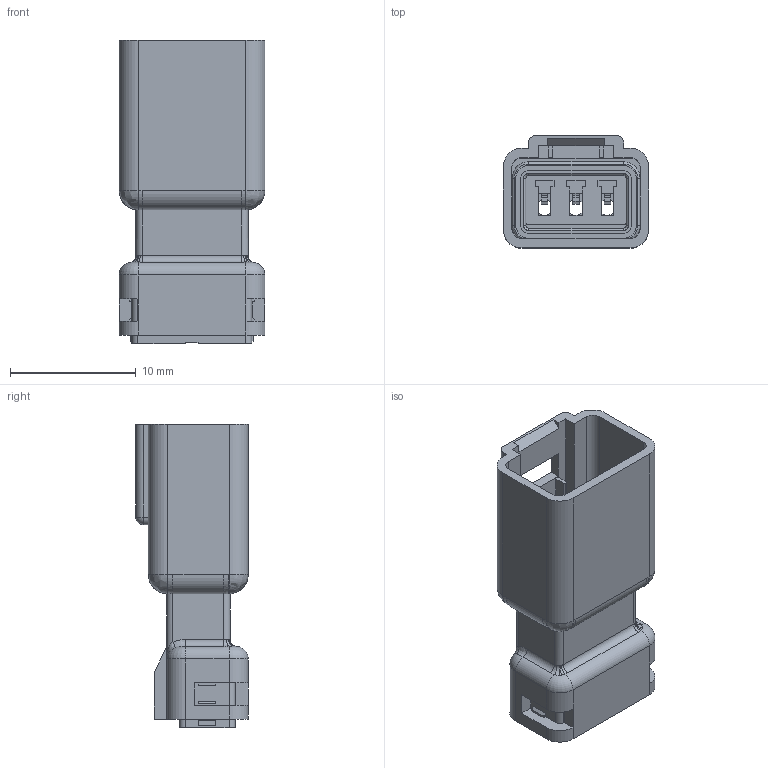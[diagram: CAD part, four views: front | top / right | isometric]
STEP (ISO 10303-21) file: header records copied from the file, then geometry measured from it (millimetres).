
FILE_DESCRIPTION (( 'STEP AP214' ), '1' );
FILE_NAME ('565-003-000-311.STEP', '2020-07-27T15:17:34', ( '' ), ( '' ), 'SwSTEP 2.0', 'SolidWorks 2020', '' );
FILE_SCHEMA (( 'AUTOMOTIVE_DESIGN' ));
Length unit declared in the file: millimetre
Products named in the file (5): 565-003-000-311_Front Gasket; 565-003-000-311; 565-003-000-311_Housing; 565-003-000-311_Rear Gasket; 565-003-000-311_Rear Insulator
Assembly tree (4 placements, depth 2):
  565-003-000-311
    565-003-000-311_Housing
    565-003-000-311_Rear Insulator
    565-003-000-311_Rear Gasket
    565-003-000-311_Front Gasket
Bounding box: 11.6 x 8.95 x 24.18 mm (x, y, z)
Volume: 1133.5 mm3; surface area: 2605.9 mm2
Topology: 7 solids, 7 shells, 530 faces, 1403 edges, 906 vertices
Faces by surface type: plane 294, cylinder 142, bspline 51, torus 41, sphere 2
Entity records: 18089 total; most frequent: CARTESIAN_POINT 4810, ORIENTED_EDGE 2794, DIRECTION 2636, EDGE_CURVE 1397, VERTEX_POINT 906, VECTOR 896, LINE 896, AXIS2_PLACEMENT_3D 870
